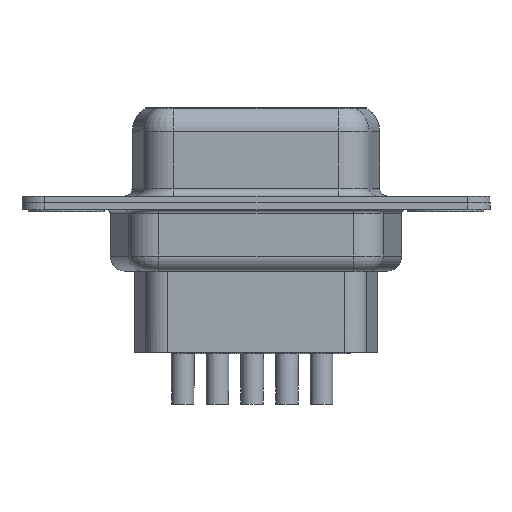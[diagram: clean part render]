
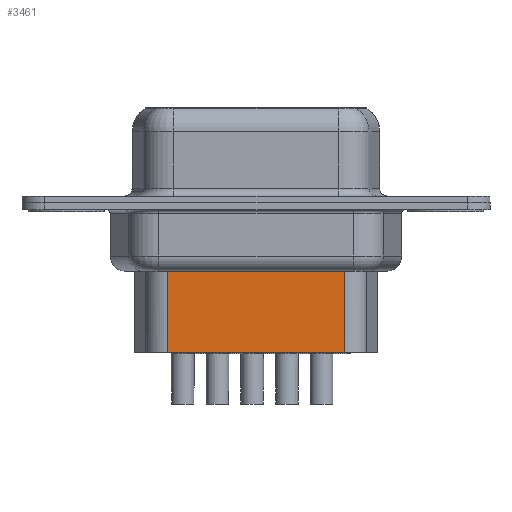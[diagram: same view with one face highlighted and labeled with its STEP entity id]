
A CAD part, front view. The second image highlights one B-rep face of the part: STEP entity #3461.
In plain terms, the highlighted planar face has unit normal (0, -1, 0).
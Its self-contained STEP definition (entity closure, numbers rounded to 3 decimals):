
#442 = EDGE_LOOP ( 'NONE', ( #18593, #15744, #19514, #16466 ) ) ;
#524 = CARTESIAN_POINT ( 'NONE',  ( 6.701, -3.5, -3.1 ) ) ;
#3012 = LINE ( 'NONE', #8871, #7783 ) ;
#3130 = VECTOR ( 'NONE', #6837, 1000. ) ;
#3461 = ADVANCED_FACE ( 'NONE', ( #10350 ), #18510, .T. ) ;
#4070 = DIRECTION ( 'NONE',  ( 0., 0., -1. ) ) ;
#5364 = DIRECTION ( 'NONE',  ( -1., 0., 0. ) ) ;
#5468 = AXIS2_PLACEMENT_3D ( 'NONE', #20470, #17701, #17364 ) ;
#5836 = EDGE_CURVE ( 'NONE', #6765, #10759, #3012, .T. ) ;
#6755 = CARTESIAN_POINT ( 'NONE',  ( 18.289, -3.5, -3.1 ) ) ;
#6765 = VERTEX_POINT ( 'NONE', #13699 ) ;
#6837 = DIRECTION ( 'NONE',  ( -1., 0., 0. ) ) ;
#7783 = VECTOR ( 'NONE', #5364, 1000. ) ;
#8871 = CARTESIAN_POINT ( 'NONE',  ( 6.701, -3.5, -9.85 ) ) ;
#9834 = CARTESIAN_POINT ( 'NONE',  ( 6.701, -3.5, -9.85 ) ) ;
#9881 = VECTOR ( 'NONE', #19081, 1000. ) ;
#10350 = FACE_OUTER_BOUND ( 'NONE', #442, .T. ) ;
#10759 = VERTEX_POINT ( 'NONE', #9834 ) ;
#12060 = LINE ( 'NONE', #22657, #3130 ) ;
#13664 = EDGE_CURVE ( 'NONE', #17173, #15808, #12060, .T. ) ;
#13699 = CARTESIAN_POINT ( 'NONE',  ( 18.289, -3.5, -9.85 ) ) ;
#14574 = LINE ( 'NONE', #6755, #9881 ) ;
#15744 = ORIENTED_EDGE ( 'NONE', *, *, #13664, .T. ) ;
#15808 = VERTEX_POINT ( 'NONE', #20353 ) ;
#16466 = ORIENTED_EDGE ( 'NONE', *, *, #5836, .F. ) ;
#17173 = VERTEX_POINT ( 'NONE', #22825 ) ;
#17364 = DIRECTION ( 'NONE',  ( 1., 0., 0. ) ) ;
#17592 = VECTOR ( 'NONE', #4070, 1000. ) ;
#17701 = DIRECTION ( 'NONE',  ( 0., -1., 0. ) ) ;
#18510 = PLANE ( 'NONE',  #5468 ) ;
#18593 = ORIENTED_EDGE ( 'NONE', *, *, #19268, .F. ) ;
#19081 = DIRECTION ( 'NONE',  ( 0., 0., -1. ) ) ;
#19268 = EDGE_CURVE ( 'NONE', #17173, #6765, #14574, .T. ) ;
#19514 = ORIENTED_EDGE ( 'NONE', *, *, #19988, .T. ) ;
#19988 = EDGE_CURVE ( 'NONE', #15808, #10759, #22748, .T. ) ;
#20353 = CARTESIAN_POINT ( 'NONE',  ( 6.701, -3.5, -4.097 ) ) ;
#20470 = CARTESIAN_POINT ( 'NONE',  ( 6.701, -3.5, -3.1 ) ) ;
#22657 = CARTESIAN_POINT ( 'NONE',  ( 6.454, -3.5, -4.097 ) ) ;
#22748 = LINE ( 'NONE', #524, #17592 ) ;
#22825 = CARTESIAN_POINT ( 'NONE',  ( 18.289, -3.5, -4.097 ) ) ;
